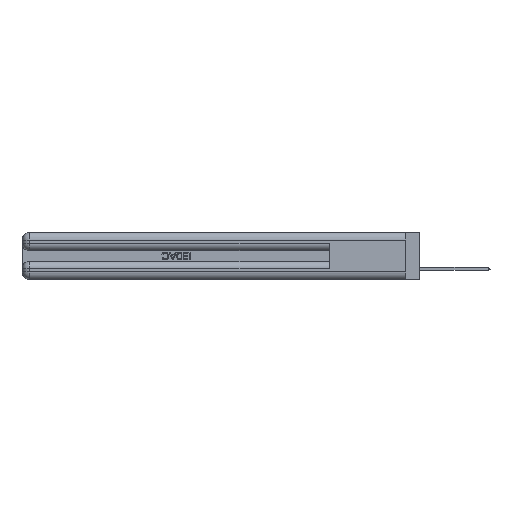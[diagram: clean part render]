
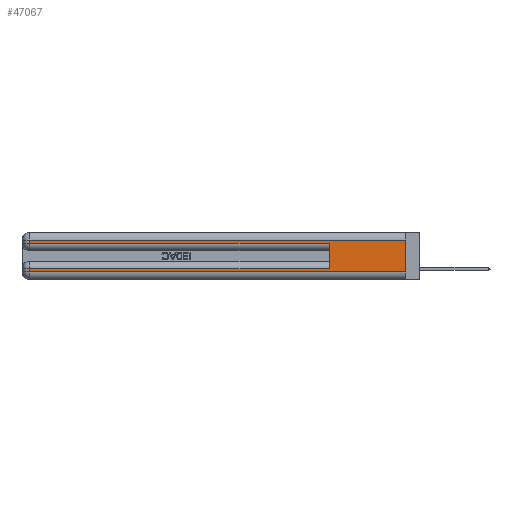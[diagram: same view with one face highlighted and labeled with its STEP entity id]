
A CAD part, left-side view. The second image highlights one B-rep face of the part: STEP entity #47067.
In plain terms, the highlighted planar face has unit normal (-1, 0, 0).
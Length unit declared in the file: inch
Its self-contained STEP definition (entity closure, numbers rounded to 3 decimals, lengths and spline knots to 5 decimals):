
#549 = PLANE ( 'NONE',  #34233 ) ;
#654 = DIRECTION ( 'NONE',  ( 0., 1., 0. ) ) ;
#1438 = LINE ( 'NONE', #31871, #13107 ) ;
#1885 = EDGE_CURVE ( 'NONE', #25756, #37419, #50614, .T. ) ;
#3514 = ORIENTED_EDGE ( 'NONE', *, *, #36459, .T. ) ;
#4284 = VECTOR ( 'NONE', #36698, 39.37008 ) ;
#4661 = DIRECTION ( 'NONE',  ( 1., 0., 0. ) ) ;
#5795 = ORIENTED_EDGE ( 'NONE', *, *, #11872, .F. ) ;
#8082 = CARTESIAN_POINT ( 'NONE',  ( 0., 0., 0.37 ) ) ;
#8834 = VERTEX_POINT ( 'NONE', #9797 ) ;
#9535 = VECTOR ( 'NONE', #11971, 39.37008 ) ;
#9797 = CARTESIAN_POINT ( 'NONE',  ( 0., 0.6, 0.085 ) ) ;
#10227 = VECTOR ( 'NONE', #654, 39.37008 ) ;
#10394 = DIRECTION ( 'NONE',  ( 0., 0., -1. ) ) ;
#11872 = EDGE_CURVE ( 'NONE', #8834, #37419, #1438, .T. ) ;
#11971 = DIRECTION ( 'NONE',  ( 0., 0., -1. ) ) ;
#12263 = VERTEX_POINT ( 'NONE', #50317 ) ;
#13107 = VECTOR ( 'NONE', #43332, 39.37008 ) ;
#14383 = LINE ( 'NONE', #15812, #28632 ) ;
#14973 = VERTEX_POINT ( 'NONE', #48719 ) ;
#15464 = FACE_OUTER_BOUND ( 'NONE', #49891, .T. ) ;
#15812 = CARTESIAN_POINT ( 'NONE',  ( 0., 0., 0.06 ) ) ;
#16842 = EDGE_CURVE ( 'NONE', #12263, #14973, #23736, .T. ) ;
#17745 = LINE ( 'NONE', #48429, #4284 ) ;
#17866 = ORIENTED_EDGE ( 'NONE', *, *, #1885, .T. ) ;
#18205 = VECTOR ( 'NONE', #36689, 39.37008 ) ;
#23736 = LINE ( 'NONE', #37950, #34920 ) ;
#23925 = DIRECTION ( 'NONE',  ( 0., -1., 0. ) ) ;
#23977 = EDGE_CURVE ( 'NONE', #8834, #12263, #17745, .T. ) ;
#24898 = LINE ( 'NONE', #47785, #9535 ) ;
#25756 = VERTEX_POINT ( 'NONE', #48067 ) ;
#28100 = CARTESIAN_POINT ( 'NONE',  ( 0., 2.94, 0.31 ) ) ;
#28632 = VECTOR ( 'NONE', #23925, 39.37008 ) ;
#30072 = LINE ( 'NONE', #31708, #10227 ) ;
#31708 = CARTESIAN_POINT ( 'NONE',  ( 0., 0., 0.31 ) ) ;
#31871 = CARTESIAN_POINT ( 'NONE',  ( 0., 0.6, 0.145 ) ) ;
#32862 = VERTEX_POINT ( 'NONE', #43158 ) ;
#33428 = EDGE_CURVE ( 'NONE', #40641, #25756, #36796, .T. ) ;
#34233 = AXIS2_PLACEMENT_3D ( 'NONE', #8082, #4661, #43726 ) ;
#34625 = ORIENTED_EDGE ( 'NONE', *, *, #33428, .T. ) ;
#34920 = VECTOR ( 'NONE', #10394, 39.37008 ) ;
#35297 = CARTESIAN_POINT ( 'NONE',  ( 0., 0., 0.285 ) ) ;
#35477 = DIRECTION ( 'NONE',  ( 0., -1., 0. ) ) ;
#36267 = VERTEX_POINT ( 'NONE', #50791 ) ;
#36459 = EDGE_CURVE ( 'NONE', #14973, #32862, #14383, .T. ) ;
#36498 = CARTESIAN_POINT ( 'NONE',  ( 0., 2.94, 0.37 ) ) ;
#36674 = ORIENTED_EDGE ( 'NONE', *, *, #45830, .F. ) ;
#36689 = DIRECTION ( 'NONE',  ( 0., 0., -1. ) ) ;
#36698 = DIRECTION ( 'NONE',  ( 0., 1., 0. ) ) ;
#36796 = LINE ( 'NONE', #36498, #18205 ) ;
#37419 = VERTEX_POINT ( 'NONE', #42097 ) ;
#37950 = CARTESIAN_POINT ( 'NONE',  ( 0., 2.94, 0.37 ) ) ;
#40641 = VERTEX_POINT ( 'NONE', #28100 ) ;
#41175 = EDGE_CURVE ( 'NONE', #36267, #40641, #30072, .T. ) ;
#42097 = CARTESIAN_POINT ( 'NONE',  ( 0., 0.6, 0.285 ) ) ;
#43158 = CARTESIAN_POINT ( 'NONE',  ( 0., 0., 0.06 ) ) ;
#43332 = DIRECTION ( 'NONE',  ( 0., 0., 1. ) ) ;
#43726 = DIRECTION ( 'NONE',  ( 0., 0., -1. ) ) ;
#45100 = ORIENTED_EDGE ( 'NONE', *, *, #16842, .T. ) ;
#45136 = VECTOR ( 'NONE', #35477, 39.37008 ) ;
#45830 = EDGE_CURVE ( 'NONE', #36267, #32862, #24898, .T. ) ;
#46818 = ORIENTED_EDGE ( 'NONE', *, *, #23977, .T. ) ;
#47067 = ADVANCED_FACE ( 'NONE', ( #15464 ), #549, .F. ) ;
#47785 = CARTESIAN_POINT ( 'NONE',  ( 0., 0., 0.37 ) ) ;
#48067 = CARTESIAN_POINT ( 'NONE',  ( 0., 2.94, 0.285 ) ) ;
#48279 = ORIENTED_EDGE ( 'NONE', *, *, #41175, .T. ) ;
#48429 = CARTESIAN_POINT ( 'NONE',  ( 0., 0., 0.085 ) ) ;
#48719 = CARTESIAN_POINT ( 'NONE',  ( 0., 2.94, 0.06 ) ) ;
#49891 = EDGE_LOOP ( 'NONE', ( #36674, #48279, #34625, #17866, #5795, #46818, #45100, #3514 ) ) ;
#50317 = CARTESIAN_POINT ( 'NONE',  ( 0., 2.94, 0.085 ) ) ;
#50614 = LINE ( 'NONE', #35297, #45136 ) ;
#50791 = CARTESIAN_POINT ( 'NONE',  ( 0., 0., 0.31 ) ) ;
